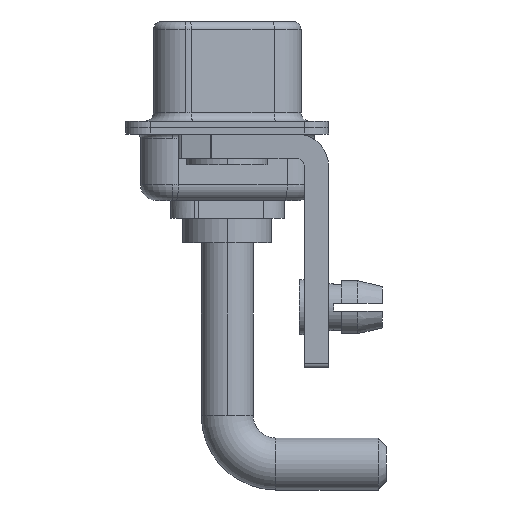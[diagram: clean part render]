
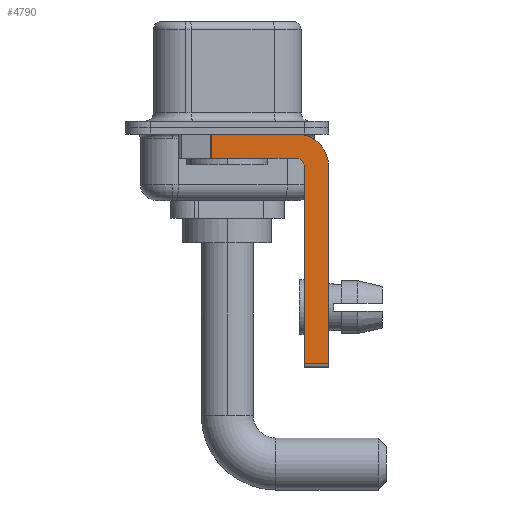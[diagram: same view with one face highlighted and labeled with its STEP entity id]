
A CAD part, left-side view. The second image highlights one B-rep face of the part: STEP entity #4790.
In plain terms, the highlighted planar face has unit normal (-1, 0, 0).
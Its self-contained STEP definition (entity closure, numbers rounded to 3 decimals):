
#308 = CARTESIAN_POINT ( 'NONE',  ( -2.9, -4.25, -1.9 ) ) ;
#527 = ORIENTED_EDGE ( 'NONE', *, *, #3931, .F. ) ;
#1444 = LINE ( 'NONE', #13136, #2569 ) ;
#1770 = EDGE_CURVE ( 'NONE', #6988, #7716, #11832, .T. ) ;
#2569 = VECTOR ( 'NONE', #14345, 1000. ) ;
#2600 = CARTESIAN_POINT ( 'NONE',  ( -2.9, 3., -0.4 ) ) ;
#2632 = VECTOR ( 'NONE', #6562, 1000. ) ;
#3220 = VERTEX_POINT ( 'NONE', #13100 ) ;
#3362 = AXIS2_PLACEMENT_3D ( 'NONE', #16729, #16909, #8210 ) ;
#3584 = DIRECTION ( 'NONE',  ( 0., 1., 0. ) ) ;
#3931 = EDGE_CURVE ( 'NONE', #3220, #6370, #16765, .T. ) ;
#4153 = LINE ( 'NONE', #11331, #10937 ) ;
#4555 = CARTESIAN_POINT ( 'NONE',  ( -2.9, 0.978, -1.9 ) ) ;
#4790 = ADVANCED_FACE ( 'NONE', ( #15325 ), #11302, .F. ) ;
#4816 = VERTEX_POINT ( 'NONE', #5622 ) ;
#5414 = LINE ( 'NONE', #2600, #18357 ) ;
#5581 = VECTOR ( 'NONE', #3584, 1000. ) ;
#5622 = CARTESIAN_POINT ( 'NONE',  ( -2.9, -6.25, -14.55 ) ) ;
#5832 = CARTESIAN_POINT ( 'NONE',  ( -2.9, -4.75, -2.4 ) ) ;
#5854 = DIRECTION ( 'NONE',  ( 0., 0., -1. ) ) ;
#6186 = VERTEX_POINT ( 'NONE', #10083 ) ;
#6370 = VERTEX_POINT ( 'NONE', #14663 ) ;
#6562 = DIRECTION ( 'NONE',  ( 0., 0., -1. ) ) ;
#6602 = EDGE_LOOP ( 'NONE', ( #13754, #9742, #14347, #10712, #15159, #16838, #15552, #527 ) ) ;
#6819 = CARTESIAN_POINT ( 'NONE',  ( -2.9, -6.25, -2.4 ) ) ;
#6985 = DIRECTION ( 'NONE',  ( -1., 0., 0. ) ) ;
#6988 = VERTEX_POINT ( 'NONE', #5832 ) ;
#7664 = AXIS2_PLACEMENT_3D ( 'NONE', #12761, #6985, #15480 ) ;
#7716 = VERTEX_POINT ( 'NONE', #10643 ) ;
#8210 = DIRECTION ( 'NONE',  ( 0., 0., -1. ) ) ;
#8282 = DIRECTION ( 'NONE',  ( 0., -1., 0. ) ) ;
#9111 = VECTOR ( 'NONE', #12678, 1000. ) ;
#9153 = EDGE_CURVE ( 'NONE', #6370, #4816, #13905, .T. ) ;
#9587 = AXIS2_PLACEMENT_3D ( 'NONE', #17049, #12838, #5854 ) ;
#9742 = ORIENTED_EDGE ( 'NONE', *, *, #13405, .T. ) ;
#9756 = EDGE_CURVE ( 'NONE', #15071, #6988, #1444, .T. ) ;
#10083 = CARTESIAN_POINT ( 'NONE',  ( -2.9, 0.978, -0.4 ) ) ;
#10357 = EDGE_CURVE ( 'NONE', #7716, #13651, #11701, .T. ) ;
#10462 = LINE ( 'NONE', #14864, #2632 ) ;
#10643 = CARTESIAN_POINT ( 'NONE',  ( -2.9, -4.25, -1.9 ) ) ;
#10712 = ORIENTED_EDGE ( 'NONE', *, *, #1770, .F. ) ;
#10937 = VECTOR ( 'NONE', #14130, 1000. ) ;
#11302 = PLANE ( 'NONE',  #3362 ) ;
#11331 = CARTESIAN_POINT ( 'NONE',  ( -2.9, -4.25, -14.55 ) ) ;
#11701 = LINE ( 'NONE', #308, #5581 ) ;
#11832 = CIRCLE ( 'NONE', #7664, 0.5 ) ;
#12678 = DIRECTION ( 'NONE',  ( 0., 0., -1. ) ) ;
#12761 = CARTESIAN_POINT ( 'NONE',  ( -2.9, -4.25, -2.4 ) ) ;
#12838 = DIRECTION ( 'NONE',  ( 1., 0., 0. ) ) ;
#13100 = CARTESIAN_POINT ( 'NONE',  ( -2.9, -4.25, -0.4 ) ) ;
#13136 = CARTESIAN_POINT ( 'NONE',  ( -2.9, -4.75, -14.8 ) ) ;
#13405 = EDGE_CURVE ( 'NONE', #6186, #13651, #10462, .T. ) ;
#13651 = VERTEX_POINT ( 'NONE', #4555 ) ;
#13754 = ORIENTED_EDGE ( 'NONE', *, *, #14248, .F. ) ;
#13905 = LINE ( 'NONE', #6819, #9111 ) ;
#14130 = DIRECTION ( 'NONE',  ( 0., -1., 0. ) ) ;
#14248 = EDGE_CURVE ( 'NONE', #6186, #3220, #5414, .T. ) ;
#14345 = DIRECTION ( 'NONE',  ( 0., 0., 1. ) ) ;
#14347 = ORIENTED_EDGE ( 'NONE', *, *, #10357, .F. ) ;
#14663 = CARTESIAN_POINT ( 'NONE',  ( -2.9, -6.25, -2.4 ) ) ;
#14864 = CARTESIAN_POINT ( 'NONE',  ( -2.9, 0.978, -1.9 ) ) ;
#15071 = VERTEX_POINT ( 'NONE', #16120 ) ;
#15159 = ORIENTED_EDGE ( 'NONE', *, *, #9756, .F. ) ;
#15325 = FACE_OUTER_BOUND ( 'NONE', #6602, .T. ) ;
#15480 = DIRECTION ( 'NONE',  ( 0., 0., 1. ) ) ;
#15552 = ORIENTED_EDGE ( 'NONE', *, *, #9153, .F. ) ;
#15750 = EDGE_CURVE ( 'NONE', #15071, #4816, #4153, .T. ) ;
#16120 = CARTESIAN_POINT ( 'NONE',  ( -2.9, -4.75, -14.55 ) ) ;
#16729 = CARTESIAN_POINT ( 'NONE',  ( -2.9, -4.25, -2.4 ) ) ;
#16765 = CIRCLE ( 'NONE', #9587, 2. ) ;
#16838 = ORIENTED_EDGE ( 'NONE', *, *, #15750, .T. ) ;
#16909 = DIRECTION ( 'NONE',  ( 1., 0., 0. ) ) ;
#17049 = CARTESIAN_POINT ( 'NONE',  ( -2.9, -4.25, -2.4 ) ) ;
#18357 = VECTOR ( 'NONE', #8282, 1000. ) ;
